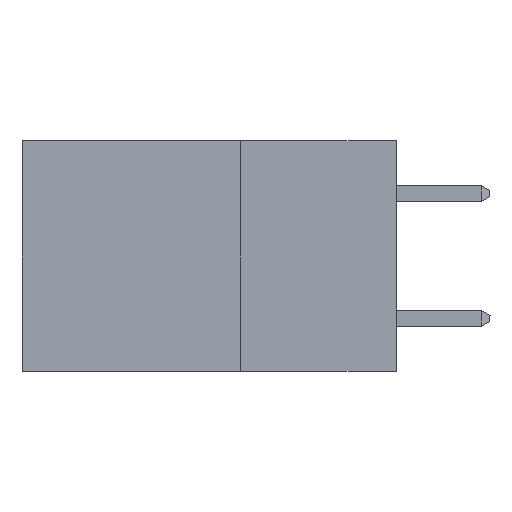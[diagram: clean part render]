
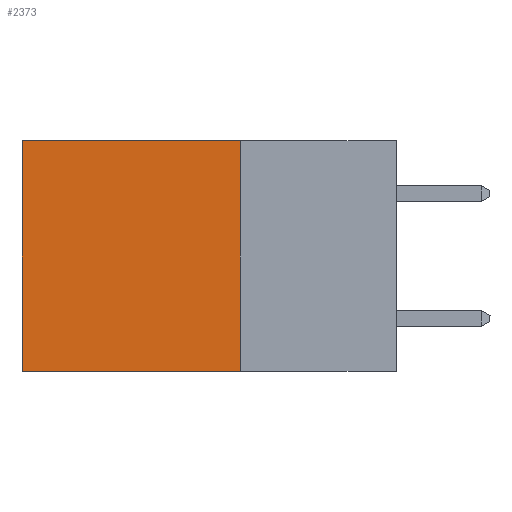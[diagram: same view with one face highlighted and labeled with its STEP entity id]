
A CAD part, left-side view. The second image highlights one B-rep face of the part: STEP entity #2373.
In plain terms, the highlighted planar face has unit normal (-1, 0, 0).
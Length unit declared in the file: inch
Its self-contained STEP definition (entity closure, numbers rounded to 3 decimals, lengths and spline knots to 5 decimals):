
#286 = AXIS2_PLACEMENT_3D ( 'NONE', #7126, #4928, #7531 ) ;
#375 = CARTESIAN_POINT ( 'NONE',  ( 0.2615, 0.6, -0.37 ) ) ;
#1483 = CARTESIAN_POINT ( 'NONE',  ( 0.2615, 0.25, 0. ) ) ;
#1663 = VECTOR ( 'NONE', #10311, 39.37008 ) ;
#1752 = CARTESIAN_POINT ( 'NONE',  ( 0.2615, 0.6, 0. ) ) ;
#1839 = ORIENTED_EDGE ( 'NONE', *, *, #8976, .F. ) ;
#2185 = VERTEX_POINT ( 'NONE', #375 ) ;
#2373 = ADVANCED_FACE ( 'NONE', ( #12098 ), #11358, .F. ) ;
#3173 = VECTOR ( 'NONE', #5392, 39.37008 ) ;
#3349 = VECTOR ( 'NONE', #4460, 39.37008 ) ;
#4460 = DIRECTION ( 'NONE',  ( 0., 0., -1. ) ) ;
#4519 = CARTESIAN_POINT ( 'NONE',  ( 0.2615, 0.6, -0.37 ) ) ;
#4724 = ORIENTED_EDGE ( 'NONE', *, *, #7408, .F. ) ;
#4776 = EDGE_LOOP ( 'NONE', ( #9641, #1839, #4724, #12239 ) ) ;
#4928 = DIRECTION ( 'NONE',  ( 1., 0., 0. ) ) ;
#5392 = DIRECTION ( 'NONE',  ( 0., 0., -1. ) ) ;
#5410 = CARTESIAN_POINT ( 'NONE',  ( 0.2615, 0.25, -0.37 ) ) ;
#5415 = VECTOR ( 'NONE', #11394, 39.37008 ) ;
#5971 = EDGE_CURVE ( 'NONE', #9157, #8077, #10242, .T. ) ;
#5991 = LINE ( 'NONE', #5410, #3173 ) ;
#6139 = LINE ( 'NONE', #4519, #3349 ) ;
#7126 = CARTESIAN_POINT ( 'NONE',  ( 0.2615, 0.25, -0.37 ) ) ;
#7408 = EDGE_CURVE ( 'NONE', #9157, #11530, #5991, .T. ) ;
#7531 = DIRECTION ( 'NONE',  ( 0., 0., -1. ) ) ;
#8077 = VERTEX_POINT ( 'NONE', #1752 ) ;
#8501 = CARTESIAN_POINT ( 'NONE',  ( 0.2615, 0.25, -0.37 ) ) ;
#8976 = EDGE_CURVE ( 'NONE', #11530, #2185, #12344, .T. ) ;
#9157 = VERTEX_POINT ( 'NONE', #1483 ) ;
#9641 = ORIENTED_EDGE ( 'NONE', *, *, #9918, .T. ) ;
#9918 = EDGE_CURVE ( 'NONE', #8077, #2185, #6139, .T. ) ;
#10242 = LINE ( 'NONE', #11339, #5415 ) ;
#10311 = DIRECTION ( 'NONE',  ( 0., 1., 0. ) ) ;
#10455 = CARTESIAN_POINT ( 'NONE',  ( 0.2615, 0.25, -0.37 ) ) ;
#11339 = CARTESIAN_POINT ( 'NONE',  ( 0.2615, 0.25, 0. ) ) ;
#11358 = PLANE ( 'NONE',  #286 ) ;
#11394 = DIRECTION ( 'NONE',  ( 0., 1., 0. ) ) ;
#11530 = VERTEX_POINT ( 'NONE', #8501 ) ;
#12098 = FACE_OUTER_BOUND ( 'NONE', #4776, .T. ) ;
#12239 = ORIENTED_EDGE ( 'NONE', *, *, #5971, .T. ) ;
#12344 = LINE ( 'NONE', #10455, #1663 ) ;
